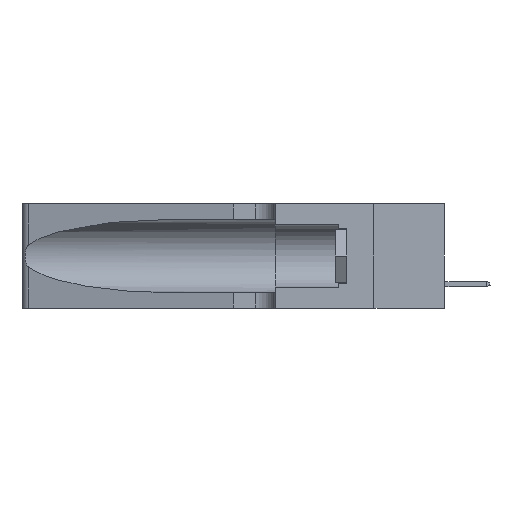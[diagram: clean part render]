
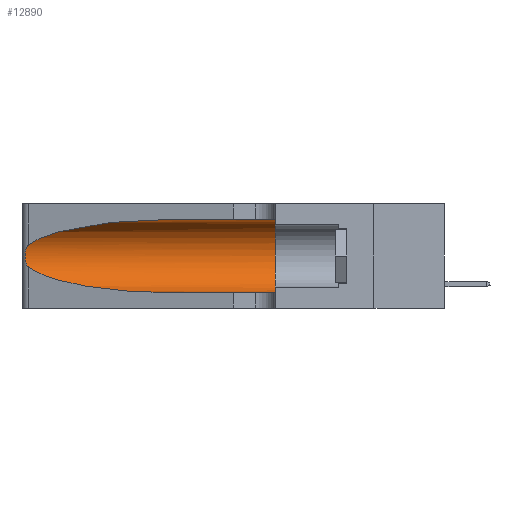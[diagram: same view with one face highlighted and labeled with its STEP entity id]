
A CAD part, left-side view. The second image highlights one B-rep face of the part: STEP entity #12890.
In plain terms, the highlighted cylindrical face has radius 3.308 mm (diameter 6.617 mm), a partial arc.
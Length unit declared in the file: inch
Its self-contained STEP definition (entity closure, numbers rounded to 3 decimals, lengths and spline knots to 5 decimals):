
#1073 = CARTESIAN_POINT ( 'NONE',  ( 0.2373, 1.15595, 0.28018 ) ) ;
#1435 = CARTESIAN_POINT ( 'NONE',  ( 0.25487, 1.22718, 0.22369 ) ) ;
#1860 = EDGE_CURVE ( 'NONE', #17151, #7220, #2990, .T. ) ;
#1909 = AXIS2_PLACEMENT_3D ( 'NONE', #16428, #18097, #14539 ) ;
#2254 = DIRECTION ( 'NONE',  ( 0., 0., -1. ) ) ;
#2674 = VERTEX_POINT ( 'NONE', #6890 ) ;
#2990 =( BOUNDED_CURVE ( )  B_SPLINE_CURVE ( 3, ( #18276, #11026, #18190, #3913 ),
 .UNSPECIFIED., .F., .T. ) 
 B_SPLINE_CURVE_WITH_KNOTS ( ( 4, 4 ),
 ( 3.44316, 4.71239 ),
 .UNSPECIFIED. ) 
 CURVE ( )  GEOMETRIC_REPRESENTATION_ITEM ( )  RATIONAL_B_SPLINE_CURVE ( ( 1., 0.87, 0.87, 1. ) ) 
 REPRESENTATION_ITEM ( '' )  );
#3036 = CARTESIAN_POINT ( 'NONE',  ( 0.25487, 1.22718, 0.22369 ) ) ;
#3077 = CARTESIAN_POINT ( 'NONE',  ( 0.25487, 1.22718, 0.14631 ) ) ;
#3834 = CARTESIAN_POINT ( 'NONE',  ( 0.1305, 0.72297, 0.31525 ) ) ;
#3913 = CARTESIAN_POINT ( 'NONE',  ( 0.1305, 0.72297, 0.05475 ) ) ;
#4819 = CARTESIAN_POINT ( 'NONE',  ( 0.26075, 1.23896, 0.19203 ) ) ;
#4916 = EDGE_CURVE ( 'NONE', #7220, #2674, #13531, .T. ) ;
#4989 = CARTESIAN_POINT ( 'NONE',  ( 0.25639, 1.23184, 0.21858 ) ) ;
#5587 = FACE_OUTER_BOUND ( 'NONE', #17075, .T. ) ;
#6586 = CARTESIAN_POINT ( 'NONE',  ( 0.25787, 1.23484, 0.2124 ) ) ;
#6743 = CARTESIAN_POINT ( 'NONE',  ( 0.25856, 1.23593, 0.16098 ) ) ;
#6847 = EDGE_CURVE ( 'NONE', #12159, #17151, #19329, .T. ) ;
#6890 = CARTESIAN_POINT ( 'NONE',  ( 0.1305, 0.35, 0.05475 ) ) ;
#7220 = VERTEX_POINT ( 'NONE', #9705 ) ;
#7719 = CARTESIAN_POINT ( 'NONE',  ( 0.1305, 0.72297, 0.31525 ) ) ;
#8075 = CIRCLE ( 'NONE', #1909, 0.13025 ) ;
#8383 = CARTESIAN_POINT ( 'NONE',  ( 0.25854, 1.2359, 0.20912 ) ) ;
#8463 = CARTESIAN_POINT ( 'NONE',  ( 0.25789, 1.23486, 0.15765 ) ) ;
#8832 = ORIENTED_EDGE ( 'NONE', *, *, #12554, .T. ) ;
#9705 = CARTESIAN_POINT ( 'NONE',  ( 0.1305, 0.72297, 0.05475 ) ) ;
#10353 = CARTESIAN_POINT ( 'NONE',  ( 0.25555, 1.22994, 0.2215 ) ) ;
#10460 = VECTOR ( 'NONE', #11029, 39.37008 ) ;
#11026 = CARTESIAN_POINT ( 'NONE',  ( 0.2373, 1.15595, 0.08982 ) ) ;
#11029 = DIRECTION ( 'NONE',  ( 0., -1., 0. ) ) ;
#11056 = ORIENTED_EDGE ( 'NONE', *, *, #4916, .T. ) ;
#12159 = VERTEX_POINT ( 'NONE', #1435 ) ;
#12329 = CYLINDRICAL_SURFACE ( 'NONE', #14335, 0.13025 ) ;
#12554 = EDGE_CURVE ( 'NONE', #16100, #12159, #15123, .T. ) ;
#12688 = VERTEX_POINT ( 'NONE', #22583 ) ;
#12890 = ADVANCED_FACE ( 'NONE', ( #5587 ), #12329, .F. ) ;
#13074 = CARTESIAN_POINT ( 'NONE',  ( 0.1305, 1.61858, 0.185 ) ) ;
#13154 = ORIENTED_EDGE ( 'NONE', *, *, #6847, .T. ) ;
#13214 = VECTOR ( 'NONE', #13582, 39.37008 ) ;
#13429 = ORIENTED_EDGE ( 'NONE', *, *, #18885, .F. ) ;
#13531 = LINE ( 'NONE', #21799, #10460 ) ;
#13582 = DIRECTION ( 'NONE',  ( 0., -1., 0. ) ) ;
#13873 = CARTESIAN_POINT ( 'NONE',  ( 0.25555, 1.22993, 0.14849 ) ) ;
#13982 = ORIENTED_EDGE ( 'NONE', *, *, #20387, .F. ) ;
#14335 = AXIS2_PLACEMENT_3D ( 'NONE', #13074, #16794, #2254 ) ;
#14539 = DIRECTION ( 'NONE',  ( 0., 0., 1. ) ) ;
#15123 =( BOUNDED_CURVE ( )  B_SPLINE_CURVE ( 3, ( #7719, #15328, #1073, #3036 ),
 .UNSPECIFIED., .F., .F. ) 
 B_SPLINE_CURVE_WITH_KNOTS ( ( 4, 4 ),
 ( 1.5708, 2.84003 ),
 .UNSPECIFIED. ) 
 CURVE ( )  GEOMETRIC_REPRESENTATION_ITEM ( )  RATIONAL_B_SPLINE_CURVE ( ( 1., 0.87, 0.87, 1. ) ) 
 REPRESENTATION_ITEM ( '' )  );
#15328 = CARTESIAN_POINT ( 'NONE',  ( 0.18966, 0.96281, 0.31525 ) ) ;
#15593 = ORIENTED_EDGE ( 'NONE', *, *, #1860, .T. ) ;
#16100 = VERTEX_POINT ( 'NONE', #3834 ) ;
#16428 = CARTESIAN_POINT ( 'NONE',  ( 0.1305, 0.35, 0.185 ) ) ;
#16794 = DIRECTION ( 'NONE',  ( 0., -1., 0. ) ) ;
#17075 = EDGE_LOOP ( 'NONE', ( #8832, #13154, #15593, #11056, #13982, #13429 ) ) ;
#17151 = VERTEX_POINT ( 'NONE', #17512 ) ;
#17357 = CARTESIAN_POINT ( 'NONE',  ( 0.25487, 1.22718, 0.22369 ) ) ;
#17438 = CARTESIAN_POINT ( 'NONE',  ( 0.26017, 1.23833, 0.17102 ) ) ;
#17512 = CARTESIAN_POINT ( 'NONE',  ( 0.25487, 1.22718, 0.14631 ) ) ;
#17549 = CARTESIAN_POINT ( 'NONE',  ( 0.1305, 1.61858, 0.31525 ) ) ;
#17597 = CARTESIAN_POINT ( 'NONE',  ( 0.26075, 1.23896, 0.178 ) ) ;
#18097 = DIRECTION ( 'NONE',  ( 0., 1., 0. ) ) ;
#18190 = CARTESIAN_POINT ( 'NONE',  ( 0.18966, 0.96281, 0.05475 ) ) ;
#18276 = CARTESIAN_POINT ( 'NONE',  ( 0.25487, 1.22718, 0.14631 ) ) ;
#18299 = LINE ( 'NONE', #17549, #13214 ) ;
#18885 = EDGE_CURVE ( 'NONE', #16100, #12688, #18299, .T. ) ;
#19329 = B_SPLINE_CURVE_WITH_KNOTS ( 'NONE', 3,
 ( #17357, #10353, #4989, #6586, #8383, #21057, #4819, #17597, #17438, #6743, #8463, #22827, #13873, #3077 ),
 .UNSPECIFIED., .F., .F.,
 ( 4, 2, 2, 2, 2, 2, 4 ),
 ( 0., 0.00027, 0.00053, 0.00107, 0.0016, 0.00187, 0.00214 ),
 .UNSPECIFIED. ) ;
#20387 = EDGE_CURVE ( 'NONE', #12688, #2674, #8075, .T. ) ;
#21057 = CARTESIAN_POINT ( 'NONE',  ( 0.26018, 1.23835, 0.19895 ) ) ;
#21799 = CARTESIAN_POINT ( 'NONE',  ( 0.1305, 1.61858, 0.05475 ) ) ;
#22583 = CARTESIAN_POINT ( 'NONE',  ( 0.1305, 0.35, 0.31525 ) ) ;
#22827 = CARTESIAN_POINT ( 'NONE',  ( 0.25639, 1.23186, 0.15144 ) ) ;
